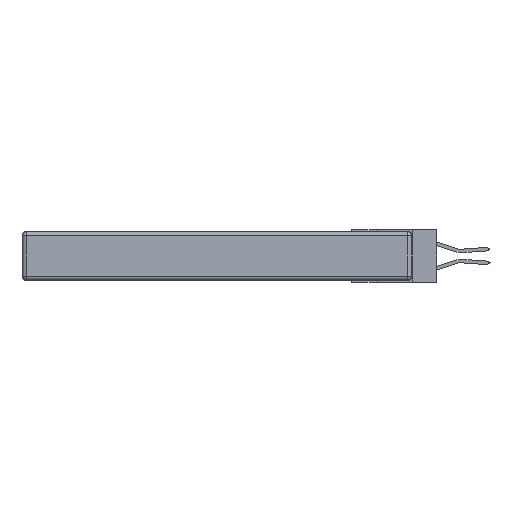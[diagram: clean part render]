
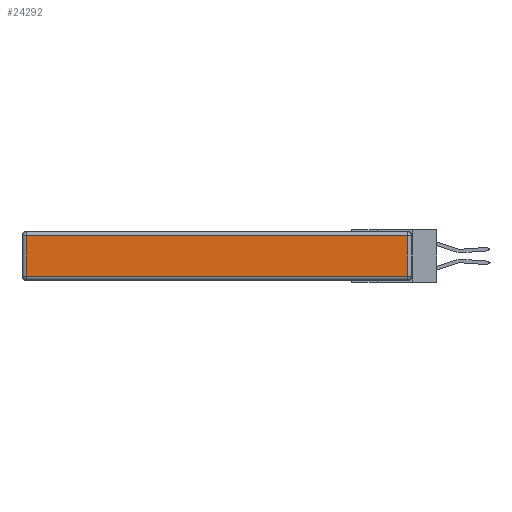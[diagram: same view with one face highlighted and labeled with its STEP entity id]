
A CAD part, left-side view. The second image highlights one B-rep face of the part: STEP entity #24292.
In plain terms, the highlighted planar face has unit normal (-1, 0, 0).
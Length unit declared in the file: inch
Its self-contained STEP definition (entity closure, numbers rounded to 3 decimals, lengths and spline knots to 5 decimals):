
#973 = DIRECTION ( 'NONE',  ( 0., 0., -1. ) ) ;
#1890 = VECTOR ( 'NONE', #973, 39.37008 ) ;
#3520 = VERTEX_POINT ( 'NONE', #27904 ) ;
#6355 = CARTESIAN_POINT ( 'NONE',  ( 0., 0.03, -0.313 ) ) ;
#6637 = CARTESIAN_POINT ( 'NONE',  ( 0., 2.72, -0.343 ) ) ;
#7423 = VERTEX_POINT ( 'NONE', #6355 ) ;
#8463 = VECTOR ( 'NONE', #23646, 39.37008 ) ;
#8719 = PLANE ( 'NONE',  #20467 ) ;
#8815 = VECTOR ( 'NONE', #26890, 39.37008 ) ;
#8842 = CARTESIAN_POINT ( 'NONE',  ( 0., 0., -0.343 ) ) ;
#8893 = VECTOR ( 'NONE', #12953, 39.37008 ) ;
#9709 = EDGE_CURVE ( 'NONE', #7423, #14125, #32939, .T. ) ;
#9971 = ORIENTED_EDGE ( 'NONE', *, *, #9709, .T. ) ;
#10251 = CARTESIAN_POINT ( 'NONE',  ( 0., 0.03, -0.343 ) ) ;
#12835 = EDGE_CURVE ( 'NONE', #19905, #3520, #26359, .T. ) ;
#12953 = DIRECTION ( 'NONE',  ( 0., 0., 1. ) ) ;
#14125 = VERTEX_POINT ( 'NONE', #30729 ) ;
#14145 = DIRECTION ( 'NONE',  ( -1., 0., 0. ) ) ;
#15306 = ORIENTED_EDGE ( 'NONE', *, *, #34009, .T. ) ;
#16843 = ORIENTED_EDGE ( 'NONE', *, *, #24658, .T. ) ;
#19905 = VERTEX_POINT ( 'NONE', #32015 ) ;
#20467 = AXIS2_PLACEMENT_3D ( 'NONE', #8842, #14145, #27802 ) ;
#23646 = DIRECTION ( 'NONE',  ( 0., 1., 0. ) ) ;
#24292 = ADVANCED_FACE ( 'NONE', ( #30848 ), #8719, .T. ) ;
#24493 = LINE ( 'NONE', #26015, #8463 ) ;
#24658 = EDGE_CURVE ( 'NONE', #14125, #19905, #24493, .T. ) ;
#26015 = CARTESIAN_POINT ( 'NONE',  ( 0., 2.75, -0.03 ) ) ;
#26359 = LINE ( 'NONE', #6637, #1890 ) ;
#26890 = DIRECTION ( 'NONE',  ( 0., -1., 0. ) ) ;
#27802 = DIRECTION ( 'NONE',  ( 0., 0., 1. ) ) ;
#27904 = CARTESIAN_POINT ( 'NONE',  ( 0., 2.72, -0.313 ) ) ;
#28224 = LINE ( 'NONE', #29828, #8815 ) ;
#29828 = CARTESIAN_POINT ( 'NONE',  ( 0., 0., -0.313 ) ) ;
#30442 = EDGE_LOOP ( 'NONE', ( #15306, #9971, #16843, #31350 ) ) ;
#30729 = CARTESIAN_POINT ( 'NONE',  ( 0., 0.03, -0.03 ) ) ;
#30848 = FACE_OUTER_BOUND ( 'NONE', #30442, .T. ) ;
#31350 = ORIENTED_EDGE ( 'NONE', *, *, #12835, .T. ) ;
#32015 = CARTESIAN_POINT ( 'NONE',  ( 0., 2.72, -0.03 ) ) ;
#32939 = LINE ( 'NONE', #10251, #8893 ) ;
#34009 = EDGE_CURVE ( 'NONE', #3520, #7423, #28224, .T. ) ;
